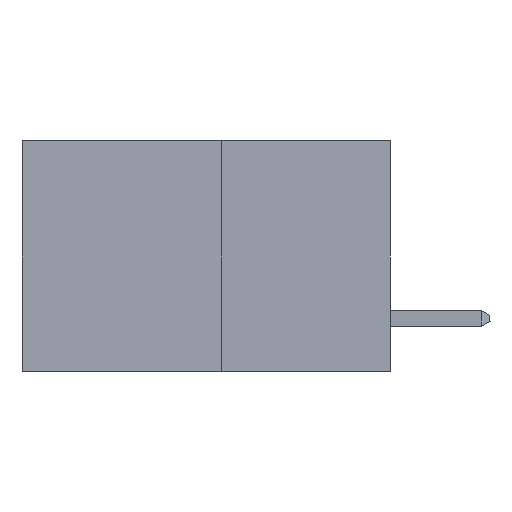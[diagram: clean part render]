
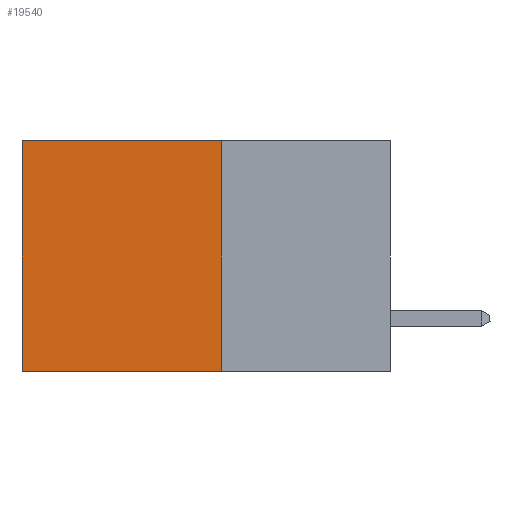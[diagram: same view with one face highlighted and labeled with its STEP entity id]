
A CAD part, left-side view. The second image highlights one B-rep face of the part: STEP entity #19540.
In plain terms, the highlighted planar face has unit normal (-1, 0, 0).
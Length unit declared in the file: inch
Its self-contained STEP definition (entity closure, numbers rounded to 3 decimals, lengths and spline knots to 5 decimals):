
#25 = EDGE_LOOP ( 'NONE', ( #13822, #30373, #29673, #28114 ) ) ;
#1461 = CARTESIAN_POINT ( 'NONE',  ( 0.277, 0.59, 0. ) ) ;
#2216 = VERTEX_POINT ( 'NONE', #23149 ) ;
#2772 = CARTESIAN_POINT ( 'NONE',  ( 0.277, 0.27, -0.37 ) ) ;
#4060 = VECTOR ( 'NONE', #28937, 39.37008 ) ;
#5251 = VERTEX_POINT ( 'NONE', #10319 ) ;
#5281 = DIRECTION ( 'NONE',  ( 0., 0., -1. ) ) ;
#5589 = DIRECTION ( 'NONE',  ( 0., 0., -1. ) ) ;
#5685 = CARTESIAN_POINT ( 'NONE',  ( 0.277, 0.27, -0.37 ) ) ;
#6410 = VECTOR ( 'NONE', #5589, 39.37008 ) ;
#6745 = CARTESIAN_POINT ( 'NONE',  ( 0.277, 0.59, -0.37 ) ) ;
#8696 = LINE ( 'NONE', #5685, #21844 ) ;
#9221 = CARTESIAN_POINT ( 'NONE',  ( 0.277, 0.27, 0. ) ) ;
#10319 = CARTESIAN_POINT ( 'NONE',  ( 0.277, 0.59, -0.37 ) ) ;
#10617 = LINE ( 'NONE', #9221, #4060 ) ;
#10622 = LINE ( 'NONE', #6745, #23743 ) ;
#12411 = VERTEX_POINT ( 'NONE', #1461 ) ;
#12597 = PLANE ( 'NONE',  #18454 ) ;
#13551 = EDGE_CURVE ( 'NONE', #2216, #5251, #8696, .T. ) ;
#13822 = ORIENTED_EDGE ( 'NONE', *, *, #21691, .T. ) ;
#15484 = DIRECTION ( 'NONE',  ( 0., 1., 0. ) ) ;
#15594 = EDGE_CURVE ( 'NONE', #23831, #12411, #10617, .T. ) ;
#18454 = AXIS2_PLACEMENT_3D ( 'NONE', #2772, #20050, #5281 ) ;
#19540 = ADVANCED_FACE ( 'NONE', ( #27360 ), #12597, .F. ) ;
#20050 = DIRECTION ( 'NONE',  ( 1., 0., 0. ) ) ;
#20357 = CARTESIAN_POINT ( 'NONE',  ( 0.277, 0.27, -0.37 ) ) ;
#21691 = EDGE_CURVE ( 'NONE', #12411, #5251, #10622, .T. ) ;
#21844 = VECTOR ( 'NONE', #15484, 39.37008 ) ;
#23149 = CARTESIAN_POINT ( 'NONE',  ( 0.277, 0.27, -0.37 ) ) ;
#23743 = VECTOR ( 'NONE', #26436, 39.37008 ) ;
#23831 = VERTEX_POINT ( 'NONE', #25211 ) ;
#25211 = CARTESIAN_POINT ( 'NONE',  ( 0.277, 0.27, 0. ) ) ;
#26436 = DIRECTION ( 'NONE',  ( 0., 0., -1. ) ) ;
#26818 = EDGE_CURVE ( 'NONE', #23831, #2216, #31805, .T. ) ;
#27360 = FACE_OUTER_BOUND ( 'NONE', #25, .T. ) ;
#28114 = ORIENTED_EDGE ( 'NONE', *, *, #15594, .T. ) ;
#28937 = DIRECTION ( 'NONE',  ( 0., 1., 0. ) ) ;
#29673 = ORIENTED_EDGE ( 'NONE', *, *, #26818, .F. ) ;
#30373 = ORIENTED_EDGE ( 'NONE', *, *, #13551, .F. ) ;
#31805 = LINE ( 'NONE', #20357, #6410 ) ;
